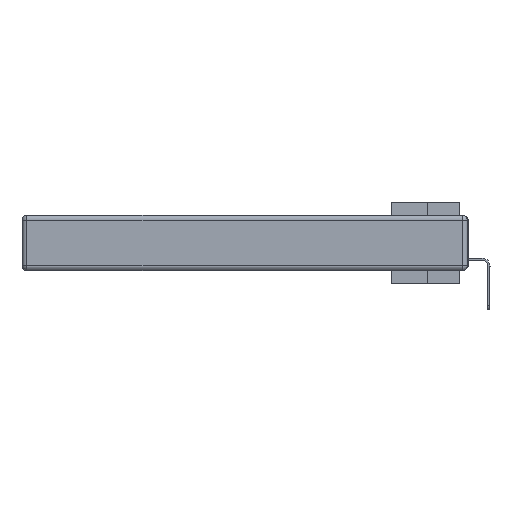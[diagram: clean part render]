
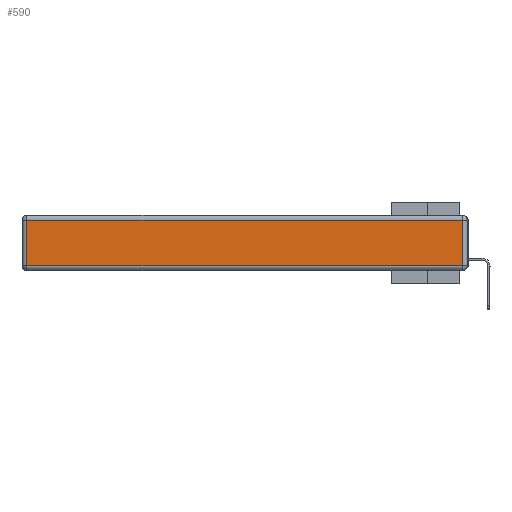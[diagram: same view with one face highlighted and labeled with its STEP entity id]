
A CAD part, left-side view. The second image highlights one B-rep face of the part: STEP entity #590.
In plain terms, the highlighted planar face has unit normal (-1, 0, 0).
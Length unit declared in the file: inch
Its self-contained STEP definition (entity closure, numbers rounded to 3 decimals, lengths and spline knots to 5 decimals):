
#590 = ADVANCED_FACE ( 'NONE', ( #31197 ), #19319, .T. ) ;
#949 = ORIENTED_EDGE ( 'NONE', *, *, #14262, .T. ) ;
#3641 = LINE ( 'NONE', #6453, #31091 ) ;
#4518 = CARTESIAN_POINT ( 'NONE',  ( 0., 0., -0.343 ) ) ;
#4586 = ORIENTED_EDGE ( 'NONE', *, *, #13255, .T. ) ;
#5878 = ORIENTED_EDGE ( 'NONE', *, *, #7795, .T. ) ;
#5928 = VERTEX_POINT ( 'NONE', #29329 ) ;
#6059 = VERTEX_POINT ( 'NONE', #25115 ) ;
#6287 = CARTESIAN_POINT ( 'NONE',  ( 0., 0.03, -0.343 ) ) ;
#6453 = CARTESIAN_POINT ( 'NONE',  ( 0., 0., -0.313 ) ) ;
#7546 = CARTESIAN_POINT ( 'NONE',  ( 0., 0.03, -0.03 ) ) ;
#7795 = EDGE_CURVE ( 'NONE', #5928, #6059, #9666, .T. ) ;
#9128 = DIRECTION ( 'NONE',  ( -1., 0., 0. ) ) ;
#9666 = LINE ( 'NONE', #16712, #21633 ) ;
#11664 = DIRECTION ( 'NONE',  ( 0., 0., 1. ) ) ;
#12655 = ORIENTED_EDGE ( 'NONE', *, *, #32589, .T. ) ;
#13255 = EDGE_CURVE ( 'NONE', #21433, #32967, #21110, .T. ) ;
#14257 = VECTOR ( 'NONE', #20909, 39.37008 ) ;
#14262 = EDGE_CURVE ( 'NONE', #32967, #5928, #17901, .T. ) ;
#16712 = CARTESIAN_POINT ( 'NONE',  ( 0., 2.72, -0.343 ) ) ;
#16944 = DIRECTION ( 'NONE',  ( 0., 0., -1. ) ) ;
#17290 = AXIS2_PLACEMENT_3D ( 'NONE', #4518, #9128, #11664 ) ;
#17901 = LINE ( 'NONE', #26221, #14257 ) ;
#18709 = VECTOR ( 'NONE', #21337, 39.37008 ) ;
#19319 = PLANE ( 'NONE',  #17290 ) ;
#20909 = DIRECTION ( 'NONE',  ( 0., 1., 0. ) ) ;
#21110 = LINE ( 'NONE', #6287, #18709 ) ;
#21337 = DIRECTION ( 'NONE',  ( 0., 0., 1. ) ) ;
#21433 = VERTEX_POINT ( 'NONE', #25488 ) ;
#21633 = VECTOR ( 'NONE', #16944, 39.37008 ) ;
#25115 = CARTESIAN_POINT ( 'NONE',  ( 0., 2.72, -0.313 ) ) ;
#25488 = CARTESIAN_POINT ( 'NONE',  ( 0., 0.03, -0.313 ) ) ;
#26221 = CARTESIAN_POINT ( 'NONE',  ( 0., 2.75, -0.03 ) ) ;
#27868 = EDGE_LOOP ( 'NONE', ( #12655, #4586, #949, #5878 ) ) ;
#29329 = CARTESIAN_POINT ( 'NONE',  ( 0., 2.72, -0.03 ) ) ;
#31091 = VECTOR ( 'NONE', #31740, 39.37008 ) ;
#31197 = FACE_OUTER_BOUND ( 'NONE', #27868, .T. ) ;
#31740 = DIRECTION ( 'NONE',  ( 0., -1., 0. ) ) ;
#32589 = EDGE_CURVE ( 'NONE', #6059, #21433, #3641, .T. ) ;
#32967 = VERTEX_POINT ( 'NONE', #7546 ) ;
